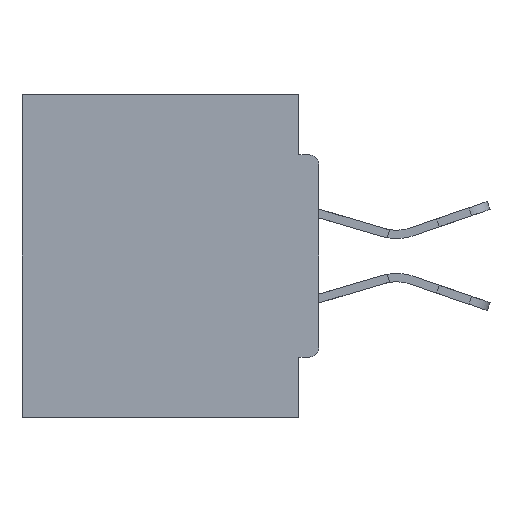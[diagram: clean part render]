
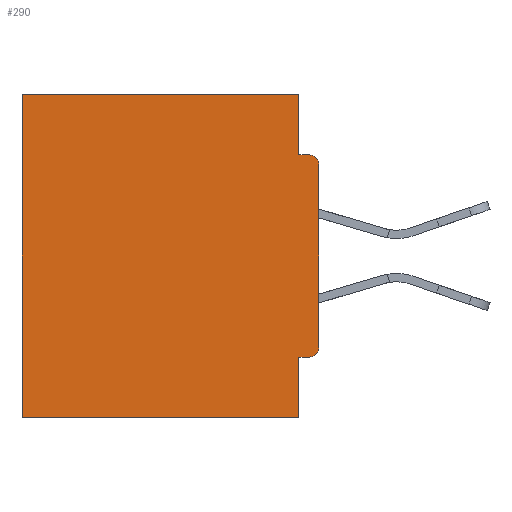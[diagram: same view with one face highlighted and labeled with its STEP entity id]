
A CAD part, left-side view. The second image highlights one B-rep face of the part: STEP entity #290.
In plain terms, the highlighted planar face has unit normal (-1, 0, 0).
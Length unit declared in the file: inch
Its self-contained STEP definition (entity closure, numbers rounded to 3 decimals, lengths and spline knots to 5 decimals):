
#85 = DIRECTION ( 'NONE',  ( 0., 0., -1. ) ) ;
#100 = CARTESIAN_POINT ( 'NONE',  ( 0.298, 0.015, -0.0935 ) ) ;
#290 = ADVANCED_FACE ( 'NONE', ( #28070 ), #25223, .F. ) ;
#1003 = ORIENTED_EDGE ( 'NONE', *, *, #14418, .F. ) ;
#1742 = LINE ( 'NONE', #7693, #3159 ) ;
#2199 = CARTESIAN_POINT ( 'NONE',  ( 0.298, 0., -0.5 ) ) ;
#2874 = EDGE_CURVE ( 'NONE', #21493, #7430, #15578, .T. ) ;
#3159 = VECTOR ( 'NONE', #17178, 39.37008 ) ;
#3319 = ORIENTED_EDGE ( 'NONE', *, *, #9350, .F. ) ;
#3425 = DIRECTION ( 'NONE',  ( -1., 0., 0. ) ) ;
#3816 = CARTESIAN_POINT ( 'NONE',  ( 0.298, 0., -0.4065 ) ) ;
#4273 = DIRECTION ( 'NONE',  ( 1., 0., 0. ) ) ;
#4409 = DIRECTION ( 'NONE',  ( 0., 0., -1. ) ) ;
#4660 = VERTEX_POINT ( 'NONE', #34044 ) ;
#5613 = VERTEX_POINT ( 'NONE', #29501 ) ;
#7430 = VERTEX_POINT ( 'NONE', #39075 ) ;
#7693 = CARTESIAN_POINT ( 'NONE',  ( 0.298, 0.46, 0. ) ) ;
#7826 = VECTOR ( 'NONE', #32437, 39.37008 ) ;
#7972 = CARTESIAN_POINT ( 'NONE',  ( 0.298, 0., 0. ) ) ;
#8377 = CARTESIAN_POINT ( 'NONE',  ( 0.298, 0.031, -0.5 ) ) ;
#8848 = VERTEX_POINT ( 'NONE', #100 ) ;
#9350 = EDGE_CURVE ( 'NONE', #20589, #4660, #19122, .T. ) ;
#9626 = EDGE_CURVE ( 'NONE', #24005, #8848, #18607, .T. ) ;
#10317 = DIRECTION ( 'NONE',  ( 0., 1., 0. ) ) ;
#10842 = DIRECTION ( 'NONE',  ( 0., 1., 0. ) ) ;
#11255 = LINE ( 'NONE', #29310, #7826 ) ;
#11508 = DIRECTION ( 'NONE',  ( 0., 0., -1. ) ) ;
#11614 = ORIENTED_EDGE ( 'NONE', *, *, #37520, .T. ) ;
#12492 = CARTESIAN_POINT ( 'NONE',  ( 0.298, 0., -0.1085 ) ) ;
#12603 = AXIS2_PLACEMENT_3D ( 'NONE', #22277, #4273, #4409 ) ;
#13081 = CARTESIAN_POINT ( 'NONE',  ( 0.298, 0.031, -0.5 ) ) ;
#13918 = DIRECTION ( 'NONE',  ( 0., 1., 0. ) ) ;
#14199 = DIRECTION ( 'NONE',  ( -1., 0., 0. ) ) ;
#14418 = EDGE_CURVE ( 'NONE', #14438, #5613, #27156, .T. ) ;
#14438 = VERTEX_POINT ( 'NONE', #29171 ) ;
#15117 = EDGE_CURVE ( 'NONE', #5613, #21493, #11255, .T. ) ;
#15578 = LINE ( 'NONE', #2199, #35897 ) ;
#15988 = EDGE_CURVE ( 'NONE', #20589, #8848, #16021, .T. ) ;
#16021 = CIRCLE ( 'NONE', #39957, 0.015 ) ;
#16531 = CARTESIAN_POINT ( 'NONE',  ( 0.298, 0., 0. ) ) ;
#16562 = VECTOR ( 'NONE', #13918, 39.37008 ) ;
#17178 = DIRECTION ( 'NONE',  ( 0., 0., -1. ) ) ;
#17756 = ORIENTED_EDGE ( 'NONE', *, *, #27327, .T. ) ;
#18237 = CARTESIAN_POINT ( 'NONE',  ( 0.298, 0., -0.0935 ) ) ;
#18607 = LINE ( 'NONE', #18237, #33581 ) ;
#19020 = ORIENTED_EDGE ( 'NONE', *, *, #15988, .T. ) ;
#19122 = LINE ( 'NONE', #7972, #25374 ) ;
#19176 = DIRECTION ( 'NONE',  ( 0., -1., 0. ) ) ;
#19319 = DIRECTION ( 'NONE',  ( 0., 0., -1. ) ) ;
#20392 = LINE ( 'NONE', #13081, #30531 ) ;
#20425 = ORIENTED_EDGE ( 'NONE', *, *, #9626, .F. ) ;
#20492 = EDGE_CURVE ( 'NONE', #21501, #37675, #25710, .T. ) ;
#20589 = VERTEX_POINT ( 'NONE', #12492 ) ;
#21493 = VERTEX_POINT ( 'NONE', #8377 ) ;
#21501 = VERTEX_POINT ( 'NONE', #24041 ) ;
#22277 = CARTESIAN_POINT ( 'NONE',  ( 0.298, 0., 0. ) ) ;
#23274 = DIRECTION ( 'NONE',  ( 0., 0., -1. ) ) ;
#24005 = VERTEX_POINT ( 'NONE', #36221 ) ;
#24041 = CARTESIAN_POINT ( 'NONE',  ( 0.298, 0.031, 0. ) ) ;
#25045 = ORIENTED_EDGE ( 'NONE', *, *, #34594, .F. ) ;
#25223 = PLANE ( 'NONE',  #12603 ) ;
#25374 = VECTOR ( 'NONE', #23274, 39.37008 ) ;
#25710 = LINE ( 'NONE', #16531, #16562 ) ;
#27020 = ORIENTED_EDGE ( 'NONE', *, *, #2874, .F. ) ;
#27156 = LINE ( 'NONE', #3816, #27646 ) ;
#27327 = EDGE_CURVE ( 'NONE', #37675, #7430, #1742, .T. ) ;
#27646 = VECTOR ( 'NONE', #10317, 39.37008 ) ;
#27904 = ORIENTED_EDGE ( 'NONE', *, *, #20492, .T. ) ;
#28070 = FACE_OUTER_BOUND ( 'NONE', #37254, .T. ) ;
#29171 = CARTESIAN_POINT ( 'NONE',  ( 0.298, 0.015, -0.4065 ) ) ;
#29310 = CARTESIAN_POINT ( 'NONE',  ( 0.298, 0.031, -0.5 ) ) ;
#29501 = CARTESIAN_POINT ( 'NONE',  ( 0.298, 0.031, -0.4065 ) ) ;
#30010 = CARTESIAN_POINT ( 'NONE',  ( 0.298, 0.015, -0.3915 ) ) ;
#30531 = VECTOR ( 'NONE', #19319, 39.37008 ) ;
#32437 = DIRECTION ( 'NONE',  ( 0., 0., -1. ) ) ;
#33581 = VECTOR ( 'NONE', #19176, 39.37008 ) ;
#34044 = CARTESIAN_POINT ( 'NONE',  ( 0.298, 0., -0.3915 ) ) ;
#34594 = EDGE_CURVE ( 'NONE', #21501, #24005, #20392, .T. ) ;
#35897 = VECTOR ( 'NONE', #10842, 39.37008 ) ;
#36221 = CARTESIAN_POINT ( 'NONE',  ( 0.298, 0.031, -0.0935 ) ) ;
#36511 = CARTESIAN_POINT ( 'NONE',  ( 0.298, 0.46, 0. ) ) ;
#36866 = AXIS2_PLACEMENT_3D ( 'NONE', #30010, #14199, #11508 ) ;
#36968 = CARTESIAN_POINT ( 'NONE',  ( 0.298, 0.015, -0.1085 ) ) ;
#37254 = EDGE_LOOP ( 'NONE', ( #19020, #20425, #25045, #27904, #17756, #27020, #38489, #1003, #11614, #3319 ) ) ;
#37520 = EDGE_CURVE ( 'NONE', #14438, #4660, #38624, .T. ) ;
#37675 = VERTEX_POINT ( 'NONE', #36511 ) ;
#38489 = ORIENTED_EDGE ( 'NONE', *, *, #15117, .F. ) ;
#38624 = CIRCLE ( 'NONE', #36866, 0.015 ) ;
#39075 = CARTESIAN_POINT ( 'NONE',  ( 0.298, 0.46, -0.5 ) ) ;
#39957 = AXIS2_PLACEMENT_3D ( 'NONE', #36968, #3425, #85 ) ;
